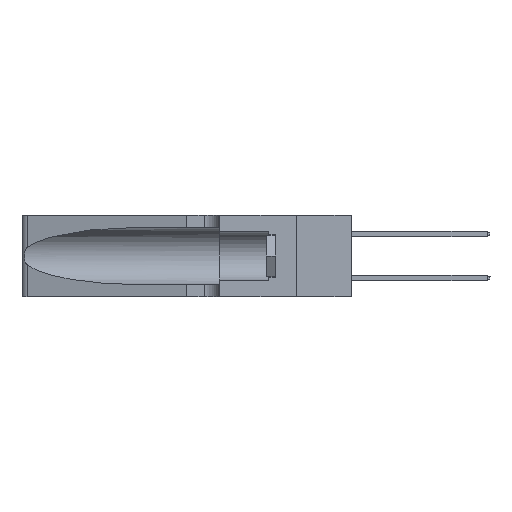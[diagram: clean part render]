
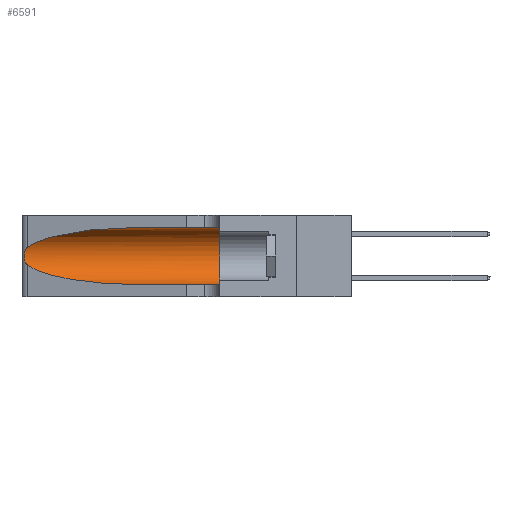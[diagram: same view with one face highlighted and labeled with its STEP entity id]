
A CAD part, left-side view. The second image highlights one B-rep face of the part: STEP entity #6591.
In plain terms, the highlighted cylindrical face has radius 3.308 mm (diameter 6.617 mm), a partial arc.
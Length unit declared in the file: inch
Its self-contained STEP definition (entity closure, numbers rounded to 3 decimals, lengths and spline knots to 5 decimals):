
#659 = ORIENTED_EDGE ( 'NONE', *, *, #3618, .F. ) ;
#924 = EDGE_LOOP ( 'NONE', ( #6511, #20150, #20415, #12315, #659, #21833 ) ) ;
#1158 = DIRECTION ( 'NONE',  ( 0., 1., 0. ) ) ;
#1323 = CARTESIAN_POINT ( 'NONE',  ( 0.25487, 1.22718, 0.14631 ) ) ;
#1509 = CARTESIAN_POINT ( 'NONE',  ( 0.1305, 0.35, 0.31525 ) ) ;
#1513 = CARTESIAN_POINT ( 'NONE',  ( 0.25639, 1.23186, 0.15144 ) ) ;
#1592 = CARTESIAN_POINT ( 'NONE',  ( 0.25555, 1.22993, 0.14849 ) ) ;
#2274 = AXIS2_PLACEMENT_3D ( 'NONE', #3252, #7204, #16951 ) ;
#2572 = CARTESIAN_POINT ( 'NONE',  ( 0.2373, 1.15595, 0.28018 ) ) ;
#2659 = CARTESIAN_POINT ( 'NONE',  ( 0.1305, 0.72297, 0.31525 ) ) ;
#2752 = CARTESIAN_POINT ( 'NONE',  ( 0.25555, 1.22994, 0.2215 ) ) ;
#3252 = CARTESIAN_POINT ( 'NONE',  ( 0.1305, 1.61858, 0.185 ) ) ;
#3485 = CARTESIAN_POINT ( 'NONE',  ( 0.25789, 1.23486, 0.15765 ) ) ;
#3618 = EDGE_CURVE ( 'NONE', #21812, #23769, #7054, .T. ) ;
#3702 = FACE_OUTER_BOUND ( 'NONE', #924, .T. ) ;
#3708 = VERTEX_POINT ( 'NONE', #1323 ) ;
#3823 =( BOUNDED_CURVE ( )  B_SPLINE_CURVE ( 3, ( #11916, #13968, #19503, #15888 ),
 .UNSPECIFIED., .F., .F. ) 
 B_SPLINE_CURVE_WITH_KNOTS ( ( 4, 4 ),
 ( 3.44316, 4.71239 ),
 .UNSPECIFIED. ) 
 CURVE ( )  GEOMETRIC_REPRESENTATION_ITEM ( )  RATIONAL_B_SPLINE_CURVE ( ( 1., 0.87, 0.87, 1. ) ) 
 REPRESENTATION_ITEM ( '' )  );
#4669 = CARTESIAN_POINT ( 'NONE',  ( 0.25854, 1.2359, 0.20912 ) ) ;
#5542 = CARTESIAN_POINT ( 'NONE',  ( 0.1305, 1.61858, 0.31525 ) ) ;
#6223 = AXIS2_PLACEMENT_3D ( 'NONE', #9080, #1158, #24110 ) ;
#6511 = ORIENTED_EDGE ( 'NONE', *, *, #8809, .T. ) ;
#6591 = ADVANCED_FACE ( 'NONE', ( #3702 ), #23433, .F. ) ;
#6942 = CARTESIAN_POINT ( 'NONE',  ( 0.25487, 1.22718, 0.22369 ) ) ;
#7054 = CIRCLE ( 'NONE', #6223, 0.13025 ) ;
#7204 = DIRECTION ( 'NONE',  ( 0., -1., 0. ) ) ;
#8177 = CARTESIAN_POINT ( 'NONE',  ( 0.1305, 0.72297, 0.05475 ) ) ;
#8481 = VERTEX_POINT ( 'NONE', #24159 ) ;
#8662 = LINE ( 'NONE', #21960, #22973 ) ;
#8809 = EDGE_CURVE ( 'NONE', #16562, #8481, #14254, .T. ) ;
#9033 = CARTESIAN_POINT ( 'NONE',  ( 0.25487, 1.22718, 0.14631 ) ) ;
#9080 = CARTESIAN_POINT ( 'NONE',  ( 0.1305, 0.35, 0.185 ) ) ;
#9903 = CARTESIAN_POINT ( 'NONE',  ( 0.1305, 0.35, 0.05475 ) ) ;
#10070 = EDGE_CURVE ( 'NONE', #10720, #23769, #8662, .T. ) ;
#10600 = DIRECTION ( 'NONE',  ( 0., -1., 0. ) ) ;
#10720 = VERTEX_POINT ( 'NONE', #8177 ) ;
#11916 = CARTESIAN_POINT ( 'NONE',  ( 0.25487, 1.22718, 0.14631 ) ) ;
#12315 = ORIENTED_EDGE ( 'NONE', *, *, #10070, .T. ) ;
#12381 = CARTESIAN_POINT ( 'NONE',  ( 0.25787, 1.23484, 0.2124 ) ) ;
#12953 = CARTESIAN_POINT ( 'NONE',  ( 0.25856, 1.23593, 0.16098 ) ) ;
#13968 = CARTESIAN_POINT ( 'NONE',  ( 0.2373, 1.15595, 0.08982 ) ) ;
#14254 =( BOUNDED_CURVE ( )  B_SPLINE_CURVE ( 3, ( #2659, #19775, #2572, #21616 ),
 .UNSPECIFIED., .F., .F. ) 
 B_SPLINE_CURVE_WITH_KNOTS ( ( 4, 4 ),
 ( 1.5708, 2.84003 ),
 .UNSPECIFIED. ) 
 CURVE ( )  GEOMETRIC_REPRESENTATION_ITEM ( )  RATIONAL_B_SPLINE_CURVE ( ( 1., 0.87, 0.87, 1. ) ) 
 REPRESENTATION_ITEM ( '' )  );
#14713 = LINE ( 'NONE', #5542, #20406 ) ;
#15005 = B_SPLINE_CURVE_WITH_KNOTS ( 'NONE', 3,
 ( #6942, #2752, #16111, #12381, #4669, #18024, #20039, #21978, #16524, #12953, #3485, #1513, #1592, #9033 ),
 .UNSPECIFIED., .F., .F.,
 ( 4, 2, 2, 2, 2, 2, 4 ),
 ( 0., 0.00027, 0.00053, 0.00107, 0.0016, 0.00187, 0.00214 ),
 .UNSPECIFIED. ) ;
#15888 = CARTESIAN_POINT ( 'NONE',  ( 0.1305, 0.72297, 0.05475 ) ) ;
#16111 = CARTESIAN_POINT ( 'NONE',  ( 0.25639, 1.23184, 0.21858 ) ) ;
#16524 = CARTESIAN_POINT ( 'NONE',  ( 0.26017, 1.23833, 0.17102 ) ) ;
#16562 = VERTEX_POINT ( 'NONE', #19593 ) ;
#16951 = DIRECTION ( 'NONE',  ( 0., 0., -1. ) ) ;
#17283 = DIRECTION ( 'NONE',  ( 0., -1., 0. ) ) ;
#18024 = CARTESIAN_POINT ( 'NONE',  ( 0.26018, 1.23835, 0.19895 ) ) ;
#18497 = EDGE_CURVE ( 'NONE', #8481, #3708, #15005, .T. ) ;
#19503 = CARTESIAN_POINT ( 'NONE',  ( 0.18966, 0.96281, 0.05475 ) ) ;
#19593 = CARTESIAN_POINT ( 'NONE',  ( 0.1305, 0.72297, 0.31525 ) ) ;
#19775 = CARTESIAN_POINT ( 'NONE',  ( 0.18966, 0.96281, 0.31525 ) ) ;
#20039 = CARTESIAN_POINT ( 'NONE',  ( 0.26075, 1.23896, 0.19203 ) ) ;
#20150 = ORIENTED_EDGE ( 'NONE', *, *, #18497, .T. ) ;
#20406 = VECTOR ( 'NONE', #17283, 39.37008 ) ;
#20415 = ORIENTED_EDGE ( 'NONE', *, *, #21043, .T. ) ;
#21043 = EDGE_CURVE ( 'NONE', #3708, #10720, #3823, .T. ) ;
#21616 = CARTESIAN_POINT ( 'NONE',  ( 0.25487, 1.22718, 0.22369 ) ) ;
#21812 = VERTEX_POINT ( 'NONE', #1509 ) ;
#21833 = ORIENTED_EDGE ( 'NONE', *, *, #24553, .F. ) ;
#21960 = CARTESIAN_POINT ( 'NONE',  ( 0.1305, 1.61858, 0.05475 ) ) ;
#21978 = CARTESIAN_POINT ( 'NONE',  ( 0.26075, 1.23896, 0.178 ) ) ;
#22973 = VECTOR ( 'NONE', #10600, 39.37008 ) ;
#23433 = CYLINDRICAL_SURFACE ( 'NONE', #2274, 0.13025 ) ;
#23769 = VERTEX_POINT ( 'NONE', #9903 ) ;
#24110 = DIRECTION ( 'NONE',  ( 0., 0., 1. ) ) ;
#24159 = CARTESIAN_POINT ( 'NONE',  ( 0.25487, 1.22718, 0.22369 ) ) ;
#24553 = EDGE_CURVE ( 'NONE', #16562, #21812, #14713, .T. ) ;
